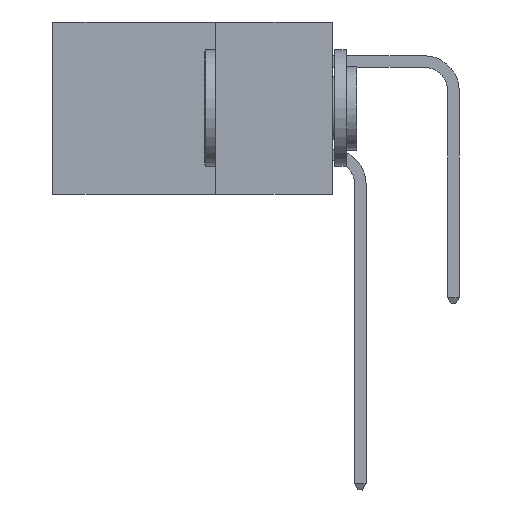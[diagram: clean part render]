
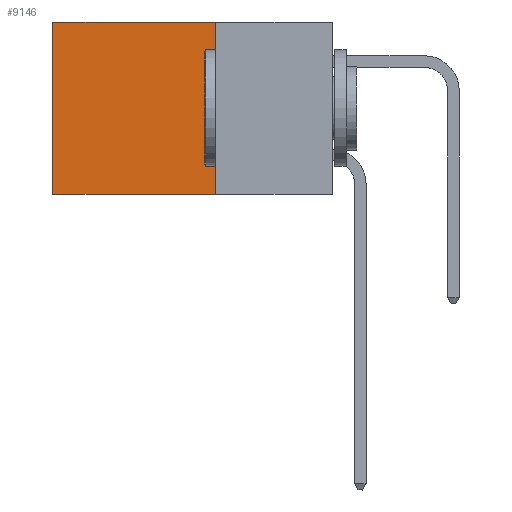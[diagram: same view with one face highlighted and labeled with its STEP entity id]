
A CAD part, left-side view. The second image highlights one B-rep face of the part: STEP entity #9146.
In plain terms, the highlighted planar face has unit normal (-1, 0, 0).
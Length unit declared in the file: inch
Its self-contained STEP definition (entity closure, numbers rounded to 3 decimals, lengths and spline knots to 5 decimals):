
#102 = VERTEX_POINT ( 'NONE', #1146 ) ;
#219 = PLANE ( 'NONE',  #18545 ) ;
#349 = CARTESIAN_POINT ( 'NONE',  ( 0.298, 0.25, -0.37 ) ) ;
#375 = DIRECTION ( 'NONE',  ( 0., 1., 0. ) ) ;
#749 = VECTOR ( 'NONE', #17462, 39.37008 ) ;
#1146 = CARTESIAN_POINT ( 'NONE',  ( 0.298, 0.25, -0.37 ) ) ;
#1572 = ORIENTED_EDGE ( 'NONE', *, *, #9031, .T. ) ;
#1684 = LINE ( 'NONE', #13148, #749 ) ;
#2268 = FACE_OUTER_BOUND ( 'NONE', #10487, .T. ) ;
#2581 = LINE ( 'NONE', #9781, #13706 ) ;
#3449 = EDGE_CURVE ( 'NONE', #102, #5283, #14394, .T. ) ;
#5283 = VERTEX_POINT ( 'NONE', #13074 ) ;
#6772 = VECTOR ( 'NONE', #11581, 39.37008 ) ;
#6818 = VECTOR ( 'NONE', #375, 39.37008 ) ;
#9031 = EDGE_CURVE ( 'NONE', #13099, #12297, #1684, .T. ) ;
#9132 = DIRECTION ( 'NONE',  ( 0., 0., -1. ) ) ;
#9146 = ADVANCED_FACE ( 'NONE', ( #2268 ), #219, .F. ) ;
#9781 = CARTESIAN_POINT ( 'NONE',  ( 0.298, 0.6, 0. ) ) ;
#10487 = EDGE_LOOP ( 'NONE', ( #16355, #18213, #14291, #1572 ) ) ;
#10549 = LINE ( 'NONE', #15816, #6772 ) ;
#11226 = DIRECTION ( 'NONE',  ( 0., 0., -1. ) ) ;
#11290 = CARTESIAN_POINT ( 'NONE',  ( 0.298, 0.6, 0. ) ) ;
#11581 = DIRECTION ( 'NONE',  ( 0., 0., -1. ) ) ;
#11943 = CARTESIAN_POINT ( 'NONE',  ( 0.298, 0.25, 0. ) ) ;
#12297 = VERTEX_POINT ( 'NONE', #11290 ) ;
#13074 = CARTESIAN_POINT ( 'NONE',  ( 0.298, 0.6, -0.37 ) ) ;
#13099 = VERTEX_POINT ( 'NONE', #15234 ) ;
#13148 = CARTESIAN_POINT ( 'NONE',  ( 0.298, 0.25, 0. ) ) ;
#13706 = VECTOR ( 'NONE', #11226, 39.37008 ) ;
#14291 = ORIENTED_EDGE ( 'NONE', *, *, #14580, .F. ) ;
#14394 = LINE ( 'NONE', #349, #6818 ) ;
#14580 = EDGE_CURVE ( 'NONE', #13099, #102, #10549, .T. ) ;
#15234 = CARTESIAN_POINT ( 'NONE',  ( 0.298, 0.25, 0. ) ) ;
#15816 = CARTESIAN_POINT ( 'NONE',  ( 0.298, 0.25, 0. ) ) ;
#16355 = ORIENTED_EDGE ( 'NONE', *, *, #18455, .T. ) ;
#17462 = DIRECTION ( 'NONE',  ( 0., 1., 0. ) ) ;
#17723 = DIRECTION ( 'NONE',  ( 1., 0., 0. ) ) ;
#18213 = ORIENTED_EDGE ( 'NONE', *, *, #3449, .F. ) ;
#18455 = EDGE_CURVE ( 'NONE', #12297, #5283, #2581, .T. ) ;
#18545 = AXIS2_PLACEMENT_3D ( 'NONE', #11943, #17723, #9132 ) ;
